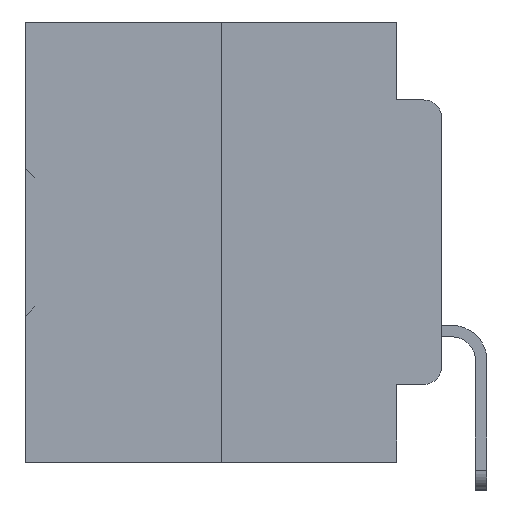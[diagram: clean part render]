
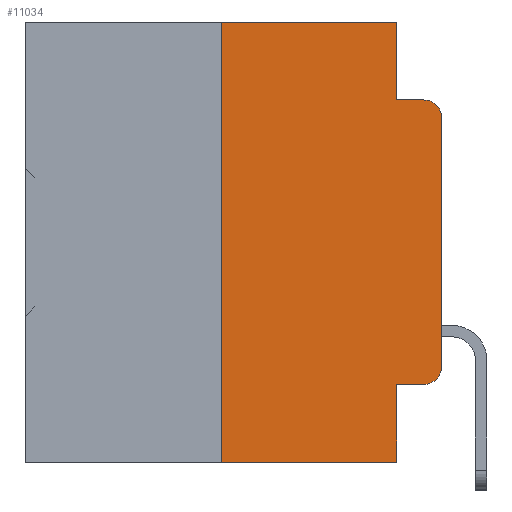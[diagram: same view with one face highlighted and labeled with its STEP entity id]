
A CAD part, left-side view. The second image highlights one B-rep face of the part: STEP entity #11034.
In plain terms, the highlighted planar face has unit normal (-1, 0, 0).
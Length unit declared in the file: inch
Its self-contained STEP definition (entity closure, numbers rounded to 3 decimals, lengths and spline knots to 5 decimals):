
#1448 = DIRECTION ( 'NONE',  ( 0., -1., 0. ) ) ;
#1751 = PLANE ( 'NONE',  #31628 ) ;
#2047 = ORIENTED_EDGE ( 'NONE', *, *, #9409, .T. ) ;
#2274 = VERTEX_POINT ( 'NONE', #37416 ) ;
#2578 = DIRECTION ( 'NONE',  ( 0., 0., -1. ) ) ;
#2805 = VERTEX_POINT ( 'NONE', #22819 ) ;
#2883 = VERTEX_POINT ( 'NONE', #23164 ) ;
#2898 = VERTEX_POINT ( 'NONE', #11236 ) ;
#3001 = DIRECTION ( 'NONE',  ( 0., 0., -1. ) ) ;
#3585 = CARTESIAN_POINT ( 'NONE',  ( 0., 0.02, -0.4115 ) ) ;
#3807 = DIRECTION ( 'NONE',  ( 0., 0., 1. ) ) ;
#4080 = VECTOR ( 'NONE', #1448, 39.37008 ) ;
#4631 = VECTOR ( 'NONE', #3807, 39.37008 ) ;
#4905 = CIRCLE ( 'NONE', #24816, 0.02 ) ;
#6023 = LINE ( 'NONE', #8949, #20874 ) ;
#6366 = EDGE_CURVE ( 'NONE', #25790, #2883, #12225, .T. ) ;
#7016 = CARTESIAN_POINT ( 'NONE',  ( 0., 0.473, -0.5 ) ) ;
#7326 = EDGE_CURVE ( 'NONE', #29336, #16717, #4905, .T. ) ;
#7411 = ORIENTED_EDGE ( 'NONE', *, *, #6366, .T. ) ;
#8021 = DIRECTION ( 'NONE',  ( 0., 0., -1. ) ) ;
#8949 = CARTESIAN_POINT ( 'NONE',  ( 0., 0.25, 0. ) ) ;
#9360 = DIRECTION ( 'NONE',  ( 0., -1., 0. ) ) ;
#9409 = EDGE_CURVE ( 'NONE', #23640, #29336, #17423, .T. ) ;
#11034 = ADVANCED_FACE ( 'NONE', ( #24506 ), #1751, .F. ) ;
#11236 = CARTESIAN_POINT ( 'NONE',  ( 0., 0.051, 0. ) ) ;
#11978 = DIRECTION ( 'NONE',  ( 0., 0., 1. ) ) ;
#12225 = LINE ( 'NONE', #7016, #26859 ) ;
#12621 = ORIENTED_EDGE ( 'NONE', *, *, #21235, .F. ) ;
#13111 = EDGE_LOOP ( 'NONE', ( #23639, #25428, #19492, #12621, #28205, #22255, #7411, #17277, #2047, #27753 ) ) ;
#13164 = CIRCLE ( 'NONE', #36282, 0.02 ) ;
#13777 = VECTOR ( 'NONE', #33778, 39.37008 ) ;
#13862 = VERTEX_POINT ( 'NONE', #17988 ) ;
#16653 = CARTESIAN_POINT ( 'NONE',  ( 0., 0.473, 0. ) ) ;
#16717 = VERTEX_POINT ( 'NONE', #24207 ) ;
#17277 = ORIENTED_EDGE ( 'NONE', *, *, #17390, .F. ) ;
#17390 = EDGE_CURVE ( 'NONE', #23640, #2883, #34383, .T. ) ;
#17423 = LINE ( 'NONE', #33985, #37276 ) ;
#17810 = LINE ( 'NONE', #24613, #4631 ) ;
#17988 = CARTESIAN_POINT ( 'NONE',  ( 0., 0.02, -0.0885 ) ) ;
#17994 = VERTEX_POINT ( 'NONE', #29205 ) ;
#19289 = EDGE_CURVE ( 'NONE', #25790, #2274, #6023, .T. ) ;
#19492 = ORIENTED_EDGE ( 'NONE', *, *, #30948, .F. ) ;
#20539 = DIRECTION ( 'NONE',  ( -1., 0., 0. ) ) ;
#20874 = VECTOR ( 'NONE', #11978, 39.37008 ) ;
#20927 = DIRECTION ( 'NONE',  ( -1., 0., 0. ) ) ;
#20972 = CARTESIAN_POINT ( 'NONE',  ( 0., 0.25, -0.5 ) ) ;
#21045 = DIRECTION ( 'NONE',  ( 0., 0., -1. ) ) ;
#21235 = EDGE_CURVE ( 'NONE', #2898, #17994, #36486, .T. ) ;
#22255 = ORIENTED_EDGE ( 'NONE', *, *, #19289, .F. ) ;
#22764 = CARTESIAN_POINT ( 'NONE',  ( 0., 0.473, 0. ) ) ;
#22819 = CARTESIAN_POINT ( 'NONE',  ( 0., 0., -0.1085 ) ) ;
#23164 = CARTESIAN_POINT ( 'NONE',  ( 0., 0.051, -0.5 ) ) ;
#23639 = ORIENTED_EDGE ( 'NONE', *, *, #34583, .T. ) ;
#23640 = VERTEX_POINT ( 'NONE', #28054 ) ;
#24050 = CARTESIAN_POINT ( 'NONE',  ( 0., 0.051, -0.0885 ) ) ;
#24207 = CARTESIAN_POINT ( 'NONE',  ( 0., 0., -0.3915 ) ) ;
#24506 = FACE_OUTER_BOUND ( 'NONE', #13111, .T. ) ;
#24613 = CARTESIAN_POINT ( 'NONE',  ( 0., 0., 0. ) ) ;
#24816 = AXIS2_PLACEMENT_3D ( 'NONE', #37762, #20927, #3001 ) ;
#25428 = ORIENTED_EDGE ( 'NONE', *, *, #32791, .T. ) ;
#25606 = DIRECTION ( 'NONE',  ( 0., -1., 0. ) ) ;
#25669 = DIRECTION ( 'NONE',  ( 1., 0., 0. ) ) ;
#25790 = VERTEX_POINT ( 'NONE', #20972 ) ;
#26859 = VECTOR ( 'NONE', #30539, 39.37008 ) ;
#26969 = VECTOR ( 'NONE', #21045, 39.37008 ) ;
#27753 = ORIENTED_EDGE ( 'NONE', *, *, #7326, .T. ) ;
#28054 = CARTESIAN_POINT ( 'NONE',  ( 0., 0.051, -0.4115 ) ) ;
#28205 = ORIENTED_EDGE ( 'NONE', *, *, #33302, .F. ) ;
#29205 = CARTESIAN_POINT ( 'NONE',  ( 0., 0.051, -0.0885 ) ) ;
#29336 = VERTEX_POINT ( 'NONE', #3585 ) ;
#29731 = CARTESIAN_POINT ( 'NONE',  ( 0., 0.051, 0. ) ) ;
#30539 = DIRECTION ( 'NONE',  ( 0., -1., 0. ) ) ;
#30948 = EDGE_CURVE ( 'NONE', #17994, #13862, #37765, .T. ) ;
#31031 = CARTESIAN_POINT ( 'NONE',  ( 0., 0.051, 0. ) ) ;
#31469 = VECTOR ( 'NONE', #9360, 39.37008 ) ;
#31628 = AXIS2_PLACEMENT_3D ( 'NONE', #22764, #25669, #8021 ) ;
#32791 = EDGE_CURVE ( 'NONE', #2805, #13862, #13164, .T. ) ;
#33302 = EDGE_CURVE ( 'NONE', #2274, #2898, #35101, .T. ) ;
#33778 = DIRECTION ( 'NONE',  ( 0., 0., -1. ) ) ;
#33985 = CARTESIAN_POINT ( 'NONE',  ( 0., 0.051, -0.4115 ) ) ;
#34383 = LINE ( 'NONE', #29731, #26969 ) ;
#34583 = EDGE_CURVE ( 'NONE', #16717, #2805, #17810, .T. ) ;
#35101 = LINE ( 'NONE', #16653, #4080 ) ;
#36282 = AXIS2_PLACEMENT_3D ( 'NONE', #37396, #20539, #2578 ) ;
#36486 = LINE ( 'NONE', #31031, #13777 ) ;
#37276 = VECTOR ( 'NONE', #25606, 39.37008 ) ;
#37396 = CARTESIAN_POINT ( 'NONE',  ( 0., 0.02, -0.1085 ) ) ;
#37416 = CARTESIAN_POINT ( 'NONE',  ( 0., 0.25, 0. ) ) ;
#37762 = CARTESIAN_POINT ( 'NONE',  ( 0., 0.02, -0.3915 ) ) ;
#37765 = LINE ( 'NONE', #24050, #31469 ) ;
